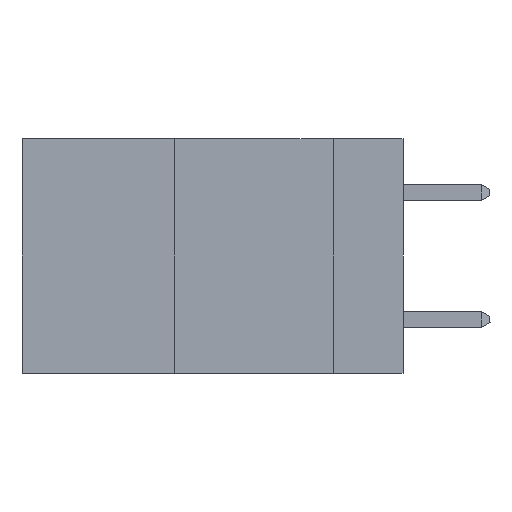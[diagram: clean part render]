
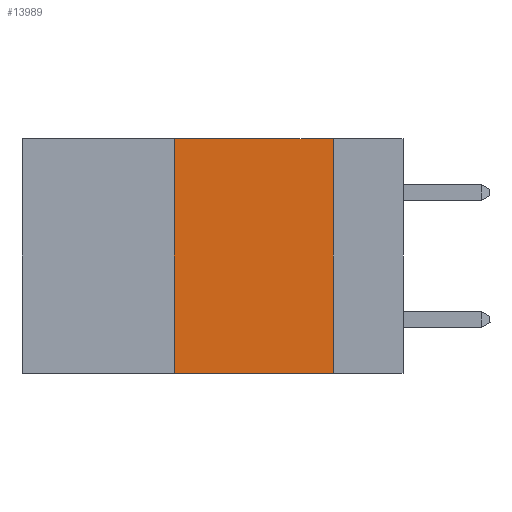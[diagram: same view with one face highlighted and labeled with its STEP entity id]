
A CAD part, left-side view. The second image highlights one B-rep face of the part: STEP entity #13989.
In plain terms, the highlighted planar face has unit normal (-1, 0, 0).
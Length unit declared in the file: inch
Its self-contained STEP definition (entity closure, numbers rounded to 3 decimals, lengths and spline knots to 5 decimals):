
#589 = EDGE_CURVE ( 'NONE', #23916, #6080, #20333, .T. ) ;
#723 = CARTESIAN_POINT ( 'NONE',  ( 0., 0.11, -0.37 ) ) ;
#3422 = VECTOR ( 'NONE', #16147, 39.37008 ) ;
#4458 = VERTEX_POINT ( 'NONE', #22993 ) ;
#5496 = DIRECTION ( 'NONE',  ( 0., -1., 0. ) ) ;
#6080 = VERTEX_POINT ( 'NONE', #12279 ) ;
#6081 = CARTESIAN_POINT ( 'NONE',  ( 0., 0.36, 0. ) ) ;
#8012 = ORIENTED_EDGE ( 'NONE', *, *, #29210, .T. ) ;
#11080 = DIRECTION ( 'NONE',  ( 0., 0., -1. ) ) ;
#11221 = VECTOR ( 'NONE', #13362, 39.37008 ) ;
#11912 = LINE ( 'NONE', #6081, #11221 ) ;
#12019 = EDGE_CURVE ( 'NONE', #4458, #23916, #11912, .T. ) ;
#12279 = CARTESIAN_POINT ( 'NONE',  ( 0., 0.11, 0. ) ) ;
#13012 = CARTESIAN_POINT ( 'NONE',  ( 0., 0.6, 0. ) ) ;
#13362 = DIRECTION ( 'NONE',  ( 0., 0., 1. ) ) ;
#13527 = PLANE ( 'NONE',  #29536 ) ;
#13989 = ADVANCED_FACE ( 'NONE', ( #28682 ), #13527, .F. ) ;
#14440 = ORIENTED_EDGE ( 'NONE', *, *, #589, .F. ) ;
#15498 = LINE ( 'NONE', #17849, #28824 ) ;
#15802 = VERTEX_POINT ( 'NONE', #723 ) ;
#16147 = DIRECTION ( 'NONE',  ( 0., -1., 0. ) ) ;
#16777 = LINE ( 'NONE', #26143, #21423 ) ;
#17849 = CARTESIAN_POINT ( 'NONE',  ( 0., 0.11, 0. ) ) ;
#18090 = EDGE_CURVE ( 'NONE', #6080, #15802, #15498, .T. ) ;
#19872 = ORIENTED_EDGE ( 'NONE', *, *, #18090, .F. ) ;
#20333 = LINE ( 'NONE', #21130, #3422 ) ;
#20453 = EDGE_LOOP ( 'NONE', ( #19872, #14440, #24986, #8012 ) ) ;
#21130 = CARTESIAN_POINT ( 'NONE',  ( 0., 0.6, 0. ) ) ;
#21423 = VECTOR ( 'NONE', #5496, 39.37008 ) ;
#22806 = CARTESIAN_POINT ( 'NONE',  ( 0., 0.36, 0. ) ) ;
#22993 = CARTESIAN_POINT ( 'NONE',  ( 0., 0.36, -0.37 ) ) ;
#23916 = VERTEX_POINT ( 'NONE', #22806 ) ;
#24986 = ORIENTED_EDGE ( 'NONE', *, *, #12019, .F. ) ;
#26143 = CARTESIAN_POINT ( 'NONE',  ( 0., 0.6, -0.37 ) ) ;
#27022 = DIRECTION ( 'NONE',  ( 0., 0., -1. ) ) ;
#27943 = DIRECTION ( 'NONE',  ( 1., 0., 0. ) ) ;
#28682 = FACE_OUTER_BOUND ( 'NONE', #20453, .T. ) ;
#28824 = VECTOR ( 'NONE', #11080, 39.37008 ) ;
#29210 = EDGE_CURVE ( 'NONE', #4458, #15802, #16777, .T. ) ;
#29536 = AXIS2_PLACEMENT_3D ( 'NONE', #13012, #27943, #27022 ) ;
